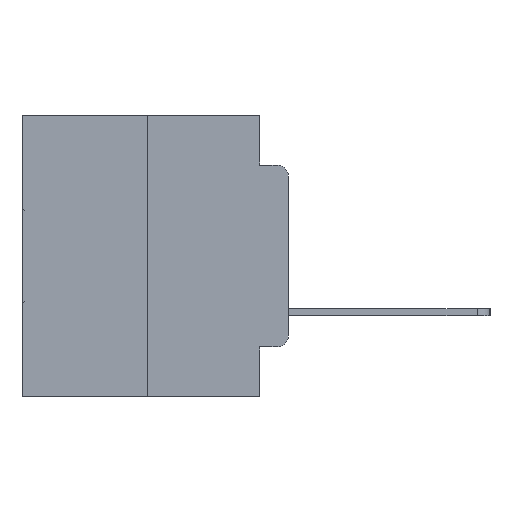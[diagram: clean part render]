
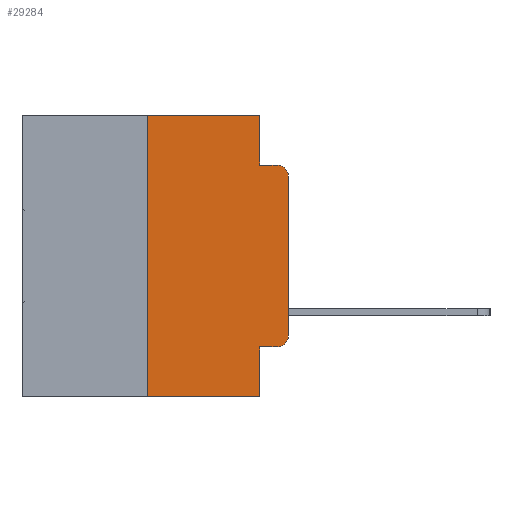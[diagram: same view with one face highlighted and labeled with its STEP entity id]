
A CAD part, left-side view. The second image highlights one B-rep face of the part: STEP entity #29284.
In plain terms, the highlighted planar face has unit normal (-1, 0, 0).
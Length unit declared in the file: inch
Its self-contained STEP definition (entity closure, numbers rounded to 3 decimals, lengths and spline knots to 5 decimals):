
#565 = CARTESIAN_POINT ( 'NONE',  ( 0., 0.473, 0. ) ) ;
#901 = LINE ( 'NONE', #7803, #5938 ) ;
#974 = LINE ( 'NONE', #22617, #16364 ) ;
#1046 = CARTESIAN_POINT ( 'NONE',  ( 0., 0.051, -0.4115 ) ) ;
#1072 = ORIENTED_EDGE ( 'NONE', *, *, #21635, .F. ) ;
#1129 = CARTESIAN_POINT ( 'NONE',  ( 0., 0.051, -0.5 ) ) ;
#1413 = ORIENTED_EDGE ( 'NONE', *, *, #17367, .T. ) ;
#1759 = VERTEX_POINT ( 'NONE', #21267 ) ;
#1803 = VERTEX_POINT ( 'NONE', #11720 ) ;
#2533 = VECTOR ( 'NONE', #2724, 39.37008 ) ;
#2554 = CARTESIAN_POINT ( 'NONE',  ( 0., 0.051, 0. ) ) ;
#2724 = DIRECTION ( 'NONE',  ( 0., -1., 0. ) ) ;
#3065 = DIRECTION ( 'NONE',  ( 0., 0., -1. ) ) ;
#3459 = VECTOR ( 'NONE', #20666, 39.37008 ) ;
#4093 = AXIS2_PLACEMENT_3D ( 'NONE', #10428, #27585, #12907 ) ;
#4222 = EDGE_CURVE ( 'NONE', #7317, #9006, #23092, .T. ) ;
#4241 = CARTESIAN_POINT ( 'NONE',  ( 0., 0.25, -0.5 ) ) ;
#5034 = DIRECTION ( 'NONE',  ( 0., 0., -1. ) ) ;
#5130 = CIRCLE ( 'NONE', #4093, 0.02 ) ;
#5430 = DIRECTION ( 'NONE',  ( 0., 0., -1. ) ) ;
#5938 = VECTOR ( 'NONE', #10135, 39.37008 ) ;
#6479 = CARTESIAN_POINT ( 'NONE',  ( 0., 0.051, -0.4115 ) ) ;
#7080 = CIRCLE ( 'NONE', #20950, 0.02 ) ;
#7105 = CARTESIAN_POINT ( 'NONE',  ( 0., 0., -0.1085 ) ) ;
#7317 = VERTEX_POINT ( 'NONE', #4241 ) ;
#7485 = CARTESIAN_POINT ( 'NONE',  ( 0., 0.473, 0. ) ) ;
#7803 = CARTESIAN_POINT ( 'NONE',  ( 0., 0.051, -0.0885 ) ) ;
#7919 = PLANE ( 'NONE',  #15183 ) ;
#8063 = VECTOR ( 'NONE', #13326, 39.37008 ) ;
#8081 = VERTEX_POINT ( 'NONE', #16990 ) ;
#8796 = CARTESIAN_POINT ( 'NONE',  ( 0., 0.25, 0. ) ) ;
#9006 = VERTEX_POINT ( 'NONE', #8796 ) ;
#9078 = LINE ( 'NONE', #7485, #2533 ) ;
#9552 = ORIENTED_EDGE ( 'NONE', *, *, #4222, .F. ) ;
#9893 = DIRECTION ( 'NONE',  ( 0., -1., 0. ) ) ;
#9898 = EDGE_CURVE ( 'NONE', #14892, #29734, #27620, .T. ) ;
#10135 = DIRECTION ( 'NONE',  ( 0., -1., 0. ) ) ;
#10390 = CARTESIAN_POINT ( 'NONE',  ( 0., 0.02, -0.3915 ) ) ;
#10428 = CARTESIAN_POINT ( 'NONE',  ( 0., 0.02, -0.1085 ) ) ;
#10903 = CARTESIAN_POINT ( 'NONE',  ( 0., 0.02, -0.4115 ) ) ;
#11434 = VECTOR ( 'NONE', #9893, 39.37008 ) ;
#11720 = CARTESIAN_POINT ( 'NONE',  ( 0., 0.02, -0.0885 ) ) ;
#12533 = VERTEX_POINT ( 'NONE', #19068 ) ;
#12642 = ORIENTED_EDGE ( 'NONE', *, *, #18271, .T. ) ;
#12811 = EDGE_CURVE ( 'NONE', #8081, #1803, #901, .T. ) ;
#12875 = DIRECTION ( 'NONE',  ( 0., 0., -1. ) ) ;
#12907 = DIRECTION ( 'NONE',  ( 0., 0., -1. ) ) ;
#13326 = DIRECTION ( 'NONE',  ( 0., -1., 0. ) ) ;
#13722 = EDGE_LOOP ( 'NONE', ( #1413, #24895, #21444, #18752, #14549, #9552, #12642, #1072, #22265, #23787 ) ) ;
#13792 = VECTOR ( 'NONE', #25214, 39.37008 ) ;
#14549 = ORIENTED_EDGE ( 'NONE', *, *, #21579, .F. ) ;
#14892 = VERTEX_POINT ( 'NONE', #6479 ) ;
#15183 = AXIS2_PLACEMENT_3D ( 'NONE', #565, #17781, #3065 ) ;
#15354 = VERTEX_POINT ( 'NONE', #7105 ) ;
#16364 = VECTOR ( 'NONE', #5430, 39.37008 ) ;
#16990 = CARTESIAN_POINT ( 'NONE',  ( 0., 0.051, -0.0885 ) ) ;
#17215 = EDGE_CURVE ( 'NONE', #12533, #8081, #29887, .T. ) ;
#17367 = EDGE_CURVE ( 'NONE', #1759, #15354, #26070, .T. ) ;
#17527 = VERTEX_POINT ( 'NONE', #1129 ) ;
#17781 = DIRECTION ( 'NONE',  ( 1., 0., 0. ) ) ;
#17813 = CARTESIAN_POINT ( 'NONE',  ( 0., 0., 0. ) ) ;
#18169 = CARTESIAN_POINT ( 'NONE',  ( 0., 0.25, 0. ) ) ;
#18271 = EDGE_CURVE ( 'NONE', #7317, #17527, #24488, .T. ) ;
#18752 = ORIENTED_EDGE ( 'NONE', *, *, #17215, .F. ) ;
#19068 = CARTESIAN_POINT ( 'NONE',  ( 0., 0.051, 0. ) ) ;
#19902 = FACE_OUTER_BOUND ( 'NONE', #13722, .T. ) ;
#20204 = EDGE_CURVE ( 'NONE', #15354, #1803, #5130, .T. ) ;
#20666 = DIRECTION ( 'NONE',  ( 0., 0., 1. ) ) ;
#20950 = AXIS2_PLACEMENT_3D ( 'NONE', #10390, #27547, #12875 ) ;
#21052 = EDGE_CURVE ( 'NONE', #29734, #1759, #7080, .T. ) ;
#21267 = CARTESIAN_POINT ( 'NONE',  ( 0., 0., -0.3915 ) ) ;
#21444 = ORIENTED_EDGE ( 'NONE', *, *, #12811, .F. ) ;
#21579 = EDGE_CURVE ( 'NONE', #9006, #12533, #9078, .T. ) ;
#21635 = EDGE_CURVE ( 'NONE', #14892, #17527, #974, .T. ) ;
#22265 = ORIENTED_EDGE ( 'NONE', *, *, #9898, .T. ) ;
#22617 = CARTESIAN_POINT ( 'NONE',  ( 0., 0.051, 0. ) ) ;
#23092 = LINE ( 'NONE', #18169, #3459 ) ;
#23420 = VECTOR ( 'NONE', #5034, 39.37008 ) ;
#23787 = ORIENTED_EDGE ( 'NONE', *, *, #21052, .T. ) ;
#24488 = LINE ( 'NONE', #27045, #11434 ) ;
#24895 = ORIENTED_EDGE ( 'NONE', *, *, #20204, .T. ) ;
#25214 = DIRECTION ( 'NONE',  ( 0., 0., 1. ) ) ;
#26070 = LINE ( 'NONE', #17813, #13792 ) ;
#27045 = CARTESIAN_POINT ( 'NONE',  ( 0., 0.473, -0.5 ) ) ;
#27547 = DIRECTION ( 'NONE',  ( -1., 0., 0. ) ) ;
#27585 = DIRECTION ( 'NONE',  ( -1., 0., 0. ) ) ;
#27620 = LINE ( 'NONE', #1046, #8063 ) ;
#29284 = ADVANCED_FACE ( 'NONE', ( #19902 ), #7919, .F. ) ;
#29734 = VERTEX_POINT ( 'NONE', #10903 ) ;
#29887 = LINE ( 'NONE', #2554, #23420 ) ;
